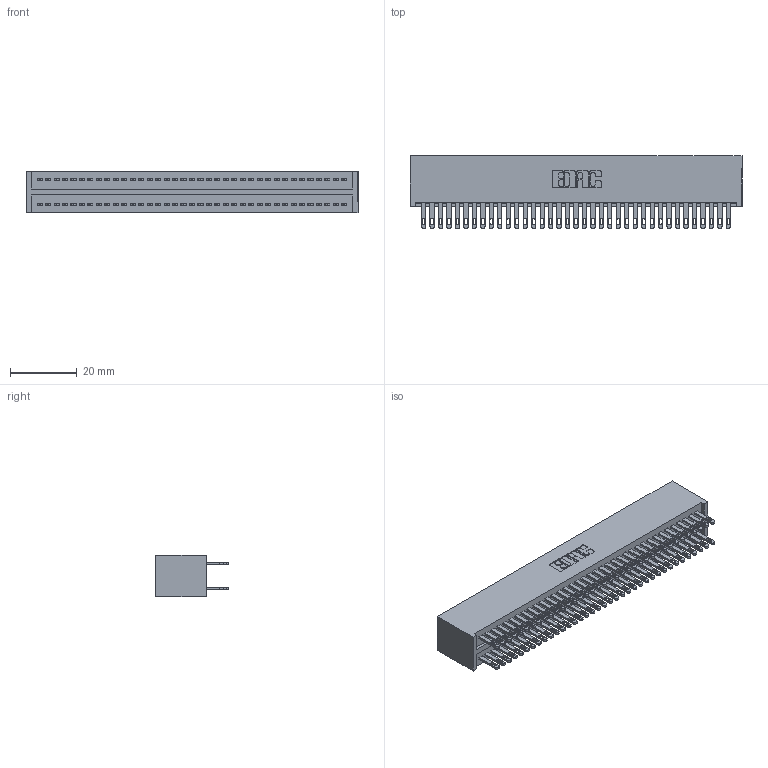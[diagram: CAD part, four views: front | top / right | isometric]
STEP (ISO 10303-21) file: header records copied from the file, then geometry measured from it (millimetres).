
FILE_DESCRIPTION (( 'STEP AP203' ), '1' );
FILE_NAME ('325-074-500-201.STEP', '2020-02-25T04:00:16', ( '' ), ( '' ), 'SwSTEP 2.0', 'SolidWorks 2016', '' );
FILE_SCHEMA (( 'CONFIG_CONTROL_DESIGN' ));
Length unit declared in the file: inch
Products named in the file (3): 325-292-001_325-293-100; 325-074-500-201; 325 Part_Lugless
Assembly tree (75 placements, depth 2):
  325-074-500-201
    325 Part_Lugless
    325-292-001_325-293-100  x74
Bounding box: 99.62 x 21.84 x 12.45 mm (x, y, z)
Volume: 13647.8 mm3; surface area: 17835.1 mm2
Topology: 75 solids, 75 shells, 3658 faces, 11165 edges, 7442 vertices
Faces by surface type: plane 2286, cylinder 1372
Entity records: 24103 total; most frequent: CARTESIAN_POINT 3998, ORIENTED_EDGE 3934, DIRECTION 3419, EDGE_CURVE 1967, VECTOR 1843, LINE 1843, VERTEX_POINT 1310, AXIS2_PLACEMENT_3D 788
